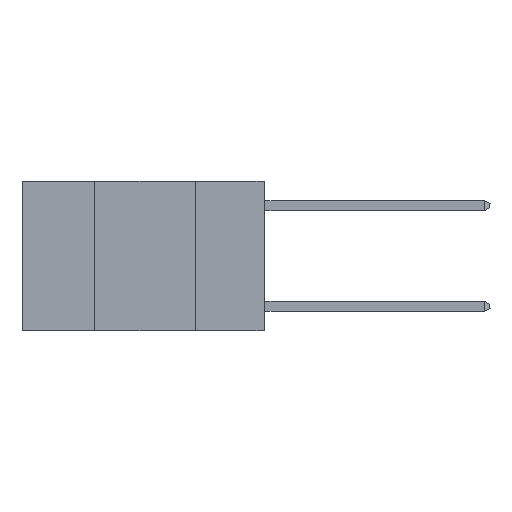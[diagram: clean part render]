
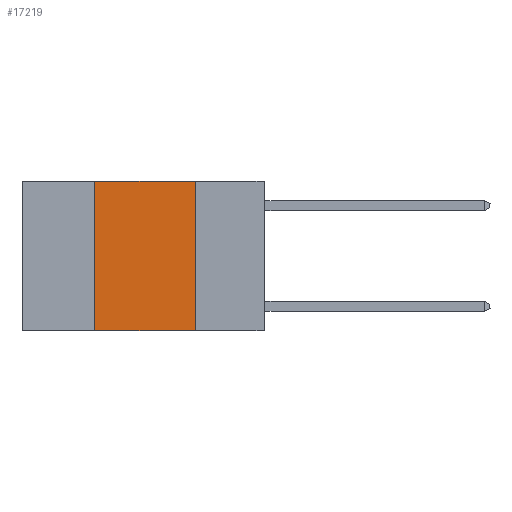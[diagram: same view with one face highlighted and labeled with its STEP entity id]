
A CAD part, left-side view. The second image highlights one B-rep face of the part: STEP entity #17219.
In plain terms, the highlighted planar face has unit normal (-1, 0, 0).
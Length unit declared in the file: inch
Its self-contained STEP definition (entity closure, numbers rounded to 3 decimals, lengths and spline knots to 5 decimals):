
#55 = AXIS2_PLACEMENT_3D ( 'NONE', #24720, #22516, #8798 ) ;
#545 = LINE ( 'NONE', #14090, #4765 ) ;
#660 = LINE ( 'NONE', #23465, #1795 ) ;
#795 = PLANE ( 'NONE',  #55 ) ;
#1095 = LINE ( 'NONE', #8970, #7831 ) ;
#1795 = VECTOR ( 'NONE', #4682, 39.37008 ) ;
#2361 = DIRECTION ( 'NONE',  ( 0., -1., 0. ) ) ;
#2968 = CARTESIAN_POINT ( 'NONE',  ( 0., 0.6, -0.37 ) ) ;
#3238 = CARTESIAN_POINT ( 'NONE',  ( 0., 0.42, 0. ) ) ;
#3609 = VECTOR ( 'NONE', #6455, 39.37008 ) ;
#4682 = DIRECTION ( 'NONE',  ( 0., 0., 1. ) ) ;
#4765 = VECTOR ( 'NONE', #2361, 39.37008 ) ;
#6455 = DIRECTION ( 'NONE',  ( 0., -1., 0. ) ) ;
#6552 = ORIENTED_EDGE ( 'NONE', *, *, #15002, .F. ) ;
#6616 = FACE_OUTER_BOUND ( 'NONE', #23020, .T. ) ;
#6888 = ORIENTED_EDGE ( 'NONE', *, *, #7956, .F. ) ;
#6936 = VERTEX_POINT ( 'NONE', #18703 ) ;
#7831 = VECTOR ( 'NONE', #14624, 39.37008 ) ;
#7956 = EDGE_CURVE ( 'NONE', #20575, #20273, #545, .T. ) ;
#8798 = DIRECTION ( 'NONE',  ( 0., 0., -1. ) ) ;
#8970 = CARTESIAN_POINT ( 'NONE',  ( 0., 0.17, 0. ) ) ;
#11854 = EDGE_CURVE ( 'NONE', #6936, #22195, #22348, .T. ) ;
#14090 = CARTESIAN_POINT ( 'NONE',  ( 0., 0.6, 0. ) ) ;
#14624 = DIRECTION ( 'NONE',  ( 0., 0., -1. ) ) ;
#15002 = EDGE_CURVE ( 'NONE', #20273, #22195, #1095, .T. ) ;
#16073 = ORIENTED_EDGE ( 'NONE', *, *, #11854, .T. ) ;
#17219 = ADVANCED_FACE ( 'NONE', ( #6616 ), #795, .F. ) ;
#18563 = CARTESIAN_POINT ( 'NONE',  ( 0., 0.17, 0. ) ) ;
#18703 = CARTESIAN_POINT ( 'NONE',  ( 0., 0.42, -0.37 ) ) ;
#19739 = ORIENTED_EDGE ( 'NONE', *, *, #21817, .F. ) ;
#20273 = VERTEX_POINT ( 'NONE', #18563 ) ;
#20575 = VERTEX_POINT ( 'NONE', #3238 ) ;
#21422 = CARTESIAN_POINT ( 'NONE',  ( 0., 0.17, -0.37 ) ) ;
#21817 = EDGE_CURVE ( 'NONE', #6936, #20575, #660, .T. ) ;
#22195 = VERTEX_POINT ( 'NONE', #21422 ) ;
#22348 = LINE ( 'NONE', #2968, #3609 ) ;
#22516 = DIRECTION ( 'NONE',  ( 1., 0., 0. ) ) ;
#23020 = EDGE_LOOP ( 'NONE', ( #6552, #6888, #19739, #16073 ) ) ;
#23465 = CARTESIAN_POINT ( 'NONE',  ( 0., 0.42, 0. ) ) ;
#24720 = CARTESIAN_POINT ( 'NONE',  ( 0., 0.6, 0. ) ) ;
